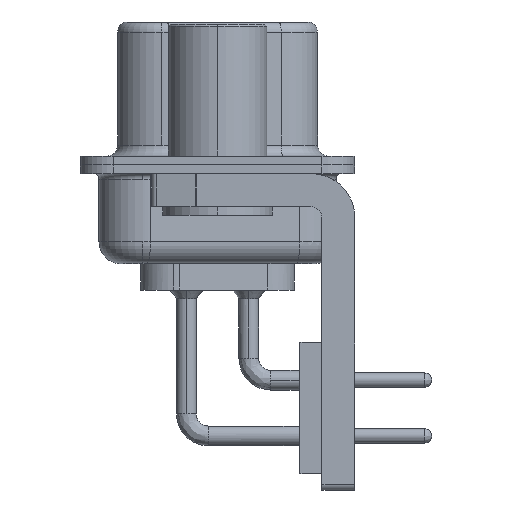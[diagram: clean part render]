
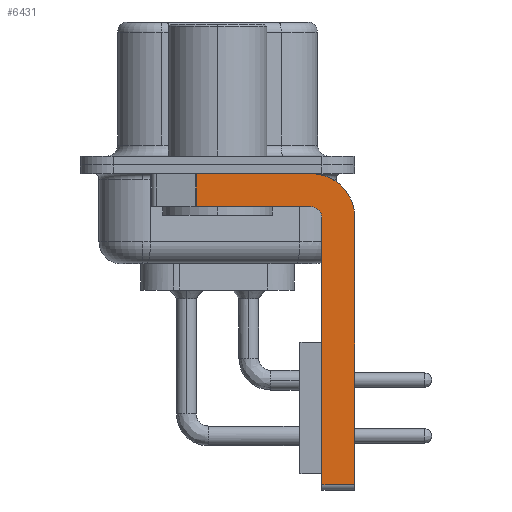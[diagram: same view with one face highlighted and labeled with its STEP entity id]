
A CAD part, left-side view. The second image highlights one B-rep face of the part: STEP entity #6431.
In plain terms, the highlighted planar face has unit normal (-1, 0, 0).
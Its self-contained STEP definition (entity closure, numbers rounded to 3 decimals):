
#2 = LINE ( 'NONE', #18810, #21149 ) ;
#93 = CARTESIAN_POINT ( 'NONE',  ( -2.9, -4.25, -0.4 ) ) ;
#330 = CARTESIAN_POINT ( 'NONE',  ( -2.9, -4.25, -1.9 ) ) ;
#347 = CARTESIAN_POINT ( 'NONE',  ( -2.9, -4.25, -2.4 ) ) ;
#1336 = CARTESIAN_POINT ( 'NONE',  ( -2.9, -4.75, -2.4 ) ) ;
#1479 = VERTEX_POINT ( 'NONE', #330 ) ;
#1999 = DIRECTION ( 'NONE',  ( 1., 0., 0. ) ) ;
#2317 = VECTOR ( 'NONE', #26323, 1000. ) ;
#2846 = LINE ( 'NONE', #20932, #27531 ) ;
#3465 = CARTESIAN_POINT ( 'NONE',  ( -2.9, 0.978, -0.4 ) ) ;
#4983 = DIRECTION ( 'NONE',  ( 0., 1., 0. ) ) ;
#6415 = CARTESIAN_POINT ( 'NONE',  ( -2.9, -4.25, -14.55 ) ) ;
#6431 = ADVANCED_FACE ( 'NONE', ( #28689 ), #29357, .F. ) ;
#6980 = CARTESIAN_POINT ( 'NONE',  ( -2.9, -6.25, -2.4 ) ) ;
#7133 = AXIS2_PLACEMENT_3D ( 'NONE', #16006, #1999, #18276 ) ;
#8106 = CARTESIAN_POINT ( 'NONE',  ( -2.9, -4.75, -14.55 ) ) ;
#8325 = VECTOR ( 'NONE', #27313, 1000. ) ;
#8409 = LINE ( 'NONE', #6415, #25472 ) ;
#8744 = DIRECTION ( 'NONE',  ( 0., -1., 0. ) ) ;
#9610 = ORIENTED_EDGE ( 'NONE', *, *, #23834, .F. ) ;
#9877 = DIRECTION ( 'NONE',  ( -1., 0., 0. ) ) ;
#9993 = ORIENTED_EDGE ( 'NONE', *, *, #26126, .T. ) ;
#10087 = CARTESIAN_POINT ( 'NONE',  ( -2.9, -4.75, -14.8 ) ) ;
#10977 = CIRCLE ( 'NONE', #7133, 2. ) ;
#11107 = AXIS2_PLACEMENT_3D ( 'NONE', #347, #29187, #28653 ) ;
#11369 = ORIENTED_EDGE ( 'NONE', *, *, #22482, .F. ) ;
#11448 = LINE ( 'NONE', #14784, #23782 ) ;
#11929 = EDGE_CURVE ( 'NONE', #19507, #26965, #11448, .T. ) ;
#12395 = VERTEX_POINT ( 'NONE', #25342 ) ;
#12474 = ORIENTED_EDGE ( 'NONE', *, *, #28407, .F. ) ;
#12626 = EDGE_CURVE ( 'NONE', #28726, #15616, #13976, .T. ) ;
#13934 = DIRECTION ( 'NONE',  ( 0., 0., -1. ) ) ;
#13976 = LINE ( 'NONE', #10087, #2317 ) ;
#14414 = ORIENTED_EDGE ( 'NONE', *, *, #12626, .F. ) ;
#14533 = LINE ( 'NONE', #24999, #8325 ) ;
#14687 = ORIENTED_EDGE ( 'NONE', *, *, #27662, .T. ) ;
#14784 = CARTESIAN_POINT ( 'NONE',  ( -2.9, 3., -0.4 ) ) ;
#14867 = CARTESIAN_POINT ( 'NONE',  ( -2.9, -6.25, -14.55 ) ) ;
#15391 = EDGE_LOOP ( 'NONE', ( #23952, #14687, #9610, #28768, #14414, #9993, #12474, #11369 ) ) ;
#15616 = VERTEX_POINT ( 'NONE', #1336 ) ;
#16006 = CARTESIAN_POINT ( 'NONE',  ( -2.9, -4.25, -2.4 ) ) ;
#16121 = CIRCLE ( 'NONE', #29211, 0.5 ) ;
#18276 = DIRECTION ( 'NONE',  ( 0., 0., -1. ) ) ;
#18810 = CARTESIAN_POINT ( 'NONE',  ( -2.9, -4.25, -1.9 ) ) ;
#19507 = VERTEX_POINT ( 'NONE', #3465 ) ;
#20932 = CARTESIAN_POINT ( 'NONE',  ( -2.9, -6.25, -2.4 ) ) ;
#21149 = VECTOR ( 'NONE', #4983, 1000. ) ;
#22184 = VERTEX_POINT ( 'NONE', #14867 ) ;
#22482 = EDGE_CURVE ( 'NONE', #26965, #25576, #10977, .T. ) ;
#23280 = EDGE_CURVE ( 'NONE', #15616, #1479, #16121, .T. ) ;
#23782 = VECTOR ( 'NONE', #28562, 1000. ) ;
#23788 = CARTESIAN_POINT ( 'NONE',  ( -2.9, -4.25, -2.4 ) ) ;
#23834 = EDGE_CURVE ( 'NONE', #1479, #12395, #2, .T. ) ;
#23952 = ORIENTED_EDGE ( 'NONE', *, *, #11929, .F. ) ;
#24999 = CARTESIAN_POINT ( 'NONE',  ( -2.9, 0.978, -1.9 ) ) ;
#25342 = CARTESIAN_POINT ( 'NONE',  ( -2.9, 0.978, -1.9 ) ) ;
#25472 = VECTOR ( 'NONE', #8744, 1000. ) ;
#25576 = VERTEX_POINT ( 'NONE', #6980 ) ;
#26095 = DIRECTION ( 'NONE',  ( 0., 0., 1. ) ) ;
#26126 = EDGE_CURVE ( 'NONE', #28726, #22184, #8409, .T. ) ;
#26323 = DIRECTION ( 'NONE',  ( 0., 0., 1. ) ) ;
#26965 = VERTEX_POINT ( 'NONE', #93 ) ;
#27313 = DIRECTION ( 'NONE',  ( 0., 0., -1. ) ) ;
#27531 = VECTOR ( 'NONE', #13934, 1000. ) ;
#27662 = EDGE_CURVE ( 'NONE', #19507, #12395, #14533, .T. ) ;
#28407 = EDGE_CURVE ( 'NONE', #25576, #22184, #2846, .T. ) ;
#28562 = DIRECTION ( 'NONE',  ( 0., -1., 0. ) ) ;
#28653 = DIRECTION ( 'NONE',  ( 0., 0., -1. ) ) ;
#28689 = FACE_OUTER_BOUND ( 'NONE', #15391, .T. ) ;
#28726 = VERTEX_POINT ( 'NONE', #8106 ) ;
#28768 = ORIENTED_EDGE ( 'NONE', *, *, #23280, .F. ) ;
#29187 = DIRECTION ( 'NONE',  ( 1., 0., 0. ) ) ;
#29211 = AXIS2_PLACEMENT_3D ( 'NONE', #23788, #9877, #26095 ) ;
#29357 = PLANE ( 'NONE',  #11107 ) ;
